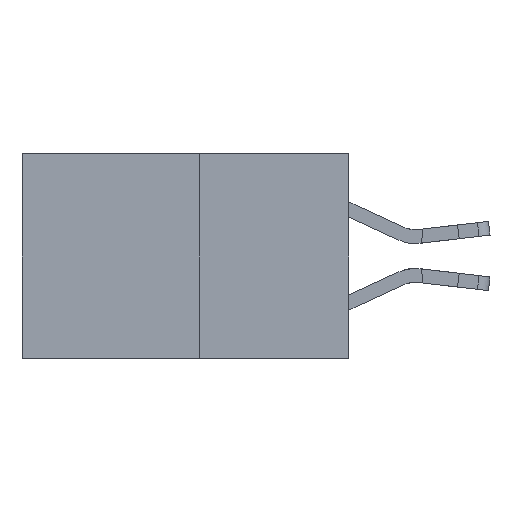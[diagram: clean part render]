
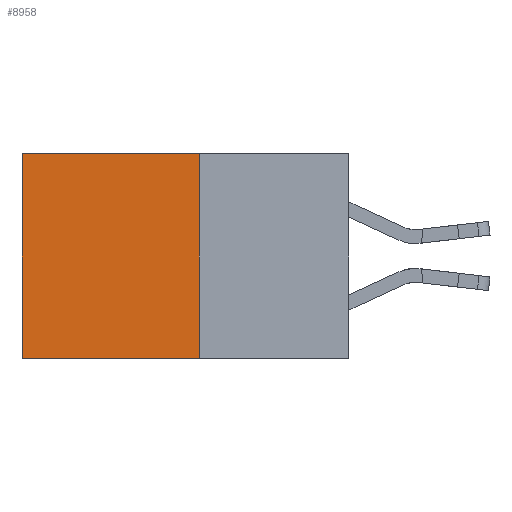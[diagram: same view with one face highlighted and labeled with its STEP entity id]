
A CAD part, left-side view. The second image highlights one B-rep face of the part: STEP entity #8958.
In plain terms, the highlighted planar face has unit normal (-1, 0, 0).
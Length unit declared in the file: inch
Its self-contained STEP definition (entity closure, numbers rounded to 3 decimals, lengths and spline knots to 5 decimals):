
#368 = LINE ( 'NONE', #21858, #17433 ) ;
#860 = LINE ( 'NONE', #3925, #5882 ) ;
#1999 = DIRECTION ( 'NONE',  ( 0., 0., -1. ) ) ;
#2100 = EDGE_CURVE ( 'NONE', #15134, #21363, #860, .T. ) ;
#2311 = CARTESIAN_POINT ( 'NONE',  ( 0.277, 0.27, -0.37 ) ) ;
#2915 = ORIENTED_EDGE ( 'NONE', *, *, #2100, .F. ) ;
#3925 = CARTESIAN_POINT ( 'NONE',  ( 0.277, 0.27, -0.37 ) ) ;
#5228 = LINE ( 'NONE', #20344, #21449 ) ;
#5585 = EDGE_LOOP ( 'NONE', ( #20337, #2915, #15685, #25586 ) ) ;
#5882 = VECTOR ( 'NONE', #6744, 39.37008 ) ;
#6185 = PLANE ( 'NONE',  #9855 ) ;
#6744 = DIRECTION ( 'NONE',  ( 0., 1., 0. ) ) ;
#7072 = DIRECTION ( 'NONE',  ( 0., 1., 0. ) ) ;
#7781 = FACE_OUTER_BOUND ( 'NONE', #5585, .T. ) ;
#8695 = DIRECTION ( 'NONE',  ( 0., 0., -1. ) ) ;
#8958 = ADVANCED_FACE ( 'NONE', ( #7781 ), #6185, .F. ) ;
#9855 = AXIS2_PLACEMENT_3D ( 'NONE', #27250, #14766, #1999 ) ;
#11183 = VECTOR ( 'NONE', #8695, 39.37008 ) ;
#11842 = LINE ( 'NONE', #2311, #11183 ) ;
#12180 = VERTEX_POINT ( 'NONE', #14817 ) ;
#13777 = EDGE_CURVE ( 'NONE', #23444, #15134, #11842, .T. ) ;
#14766 = DIRECTION ( 'NONE',  ( 1., 0., 0. ) ) ;
#14817 = CARTESIAN_POINT ( 'NONE',  ( 0.277, 0.59, 0. ) ) ;
#15005 = CARTESIAN_POINT ( 'NONE',  ( 0.277, 0.27, -0.37 ) ) ;
#15134 = VERTEX_POINT ( 'NONE', #15005 ) ;
#15685 = ORIENTED_EDGE ( 'NONE', *, *, #13777, .F. ) ;
#17433 = VECTOR ( 'NONE', #7072, 39.37008 ) ;
#19758 = CARTESIAN_POINT ( 'NONE',  ( 0.277, 0.59, -0.37 ) ) ;
#20337 = ORIENTED_EDGE ( 'NONE', *, *, #25104, .T. ) ;
#20344 = CARTESIAN_POINT ( 'NONE',  ( 0.277, 0.59, -0.37 ) ) ;
#21352 = EDGE_CURVE ( 'NONE', #23444, #12180, #368, .T. ) ;
#21363 = VERTEX_POINT ( 'NONE', #19758 ) ;
#21449 = VECTOR ( 'NONE', #26585, 39.37008 ) ;
#21858 = CARTESIAN_POINT ( 'NONE',  ( 0.277, 0.27, 0. ) ) ;
#22887 = CARTESIAN_POINT ( 'NONE',  ( 0.277, 0.27, 0. ) ) ;
#23444 = VERTEX_POINT ( 'NONE', #22887 ) ;
#25104 = EDGE_CURVE ( 'NONE', #12180, #21363, #5228, .T. ) ;
#25586 = ORIENTED_EDGE ( 'NONE', *, *, #21352, .T. ) ;
#26585 = DIRECTION ( 'NONE',  ( 0., 0., -1. ) ) ;
#27250 = CARTESIAN_POINT ( 'NONE',  ( 0.277, 0.27, -0.37 ) ) ;
